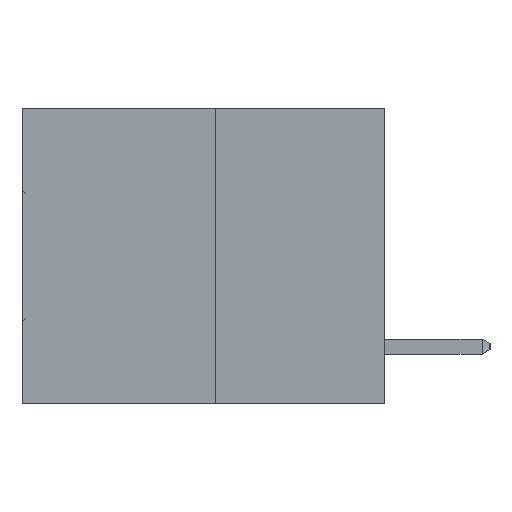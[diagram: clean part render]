
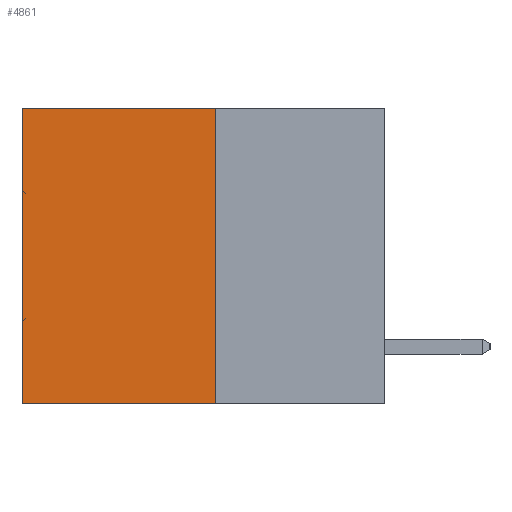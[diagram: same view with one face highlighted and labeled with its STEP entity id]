
A CAD part, left-side view. The second image highlights one B-rep face of the part: STEP entity #4861.
In plain terms, the highlighted planar face has unit normal (-1, 0, 0).
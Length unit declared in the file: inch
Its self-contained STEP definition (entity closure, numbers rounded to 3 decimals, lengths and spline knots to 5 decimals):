
#3642 = ORIENTED_EDGE ( 'NONE', *, *, #5542, .F. ) ;
#4795 = EDGE_CURVE ( 'NONE', #12940, #13123, #10594, .T. ) ;
#4861 = ADVANCED_FACE ( 'NONE', ( #12188 ), #28932, .F. ) ;
#5542 = EDGE_CURVE ( 'NONE', #6320, #13123, #6775, .T. ) ;
#6320 = VERTEX_POINT ( 'NONE', #22672 ) ;
#6618 = EDGE_LOOP ( 'NONE', ( #19320, #3642, #18164, #11528 ) ) ;
#6712 = CARTESIAN_POINT ( 'NONE',  ( 0.3165, 0.28, -0.49 ) ) ;
#6775 = LINE ( 'NONE', #16678, #17513 ) ;
#10041 = CARTESIAN_POINT ( 'NONE',  ( 0.3165, 0.28, 0. ) ) ;
#10594 = LINE ( 'NONE', #26775, #25270 ) ;
#11086 = VECTOR ( 'NONE', #13828, 39.37008 ) ;
#11528 = ORIENTED_EDGE ( 'NONE', *, *, #12655, .T. ) ;
#12188 = FACE_OUTER_BOUND ( 'NONE', #6618, .T. ) ;
#12655 = EDGE_CURVE ( 'NONE', #24567, #12940, #28848, .T. ) ;
#12940 = VERTEX_POINT ( 'NONE', #14040 ) ;
#13123 = VERTEX_POINT ( 'NONE', #20033 ) ;
#13828 = DIRECTION ( 'NONE',  ( 0., 0., -1. ) ) ;
#14040 = CARTESIAN_POINT ( 'NONE',  ( 0.3165, 0.6, 0. ) ) ;
#14388 = DIRECTION ( 'NONE',  ( 0., 0., -1. ) ) ;
#15057 = DIRECTION ( 'NONE',  ( 0., 1., 0. ) ) ;
#16678 = CARTESIAN_POINT ( 'NONE',  ( 0.3165, 0.28, -0.49 ) ) ;
#17513 = VECTOR ( 'NONE', #19119, 39.37008 ) ;
#18164 = ORIENTED_EDGE ( 'NONE', *, *, #19718, .F. ) ;
#19119 = DIRECTION ( 'NONE',  ( 0., 1., 0. ) ) ;
#19320 = ORIENTED_EDGE ( 'NONE', *, *, #4795, .T. ) ;
#19718 = EDGE_CURVE ( 'NONE', #24567, #6320, #25381, .T. ) ;
#20033 = CARTESIAN_POINT ( 'NONE',  ( 0.3165, 0.6, -0.49 ) ) ;
#20577 = CARTESIAN_POINT ( 'NONE',  ( 0.3165, 0.28, 0. ) ) ;
#21618 = DIRECTION ( 'NONE',  ( 0., 0., -1. ) ) ;
#22118 = VECTOR ( 'NONE', #15057, 39.37008 ) ;
#22672 = CARTESIAN_POINT ( 'NONE',  ( 0.3165, 0.28, -0.49 ) ) ;
#23823 = CARTESIAN_POINT ( 'NONE',  ( 0.3165, 0.28, -0.49 ) ) ;
#23947 = AXIS2_PLACEMENT_3D ( 'NONE', #6712, #32234, #14388 ) ;
#24567 = VERTEX_POINT ( 'NONE', #20577 ) ;
#25270 = VECTOR ( 'NONE', #21618, 39.37008 ) ;
#25381 = LINE ( 'NONE', #23823, #11086 ) ;
#26775 = CARTESIAN_POINT ( 'NONE',  ( 0.3165, 0.6, -0.49 ) ) ;
#28848 = LINE ( 'NONE', #10041, #22118 ) ;
#28932 = PLANE ( 'NONE',  #23947 ) ;
#32234 = DIRECTION ( 'NONE',  ( 1., 0., 0. ) ) ;
